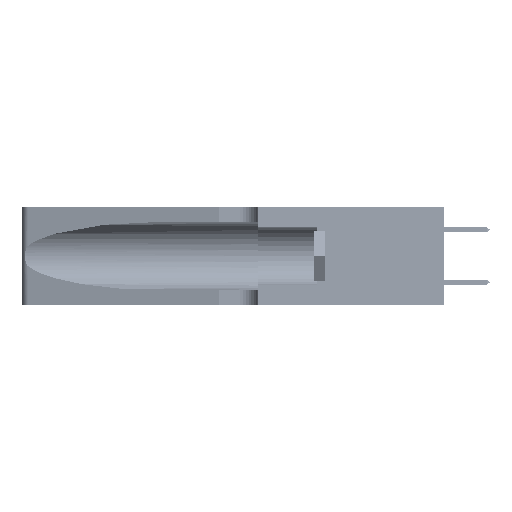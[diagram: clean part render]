
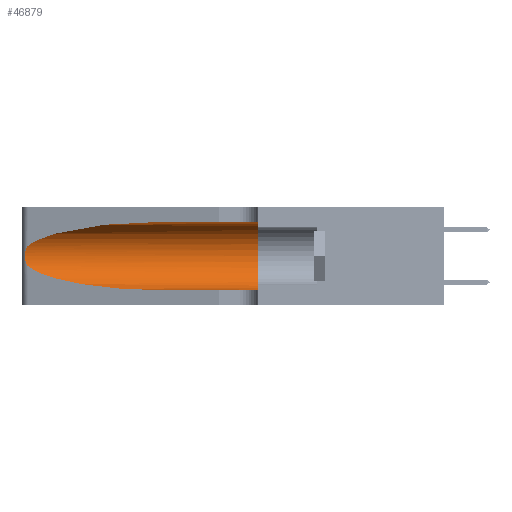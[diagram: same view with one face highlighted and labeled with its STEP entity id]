
A CAD part, left-side view. The second image highlights one B-rep face of the part: STEP entity #46879.
In plain terms, the highlighted cylindrical face has radius 3.308 mm (diameter 6.617 mm), a partial arc.
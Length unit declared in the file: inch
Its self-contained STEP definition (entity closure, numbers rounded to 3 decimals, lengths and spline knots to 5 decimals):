
#2555 = EDGE_CURVE ( 'NONE', #33973, #48274, #9177, .T. ) ;
#2716 = DIRECTION ( 'NONE',  ( 0., 1., 0. ) ) ;
#3169 = CARTESIAN_POINT ( 'NONE',  ( 0.26075, 1.23896, 0.19203 ) ) ;
#3347 = CARTESIAN_POINT ( 'NONE',  ( 0.25854, 1.2359, 0.20912 ) ) ;
#4081 = CARTESIAN_POINT ( 'NONE',  ( 0.25487, 1.22718, 0.14631 ) ) ;
#6239 = CARTESIAN_POINT ( 'NONE',  ( 0.2373, 1.15595, 0.08982 ) ) ;
#6673 = CARTESIAN_POINT ( 'NONE',  ( 0.25487, 1.22718, 0.22369 ) ) ;
#7035 = ORIENTED_EDGE ( 'NONE', *, *, #21772, .T. ) ;
#7107 = VERTEX_POINT ( 'NONE', #26929 ) ;
#7726 = CARTESIAN_POINT ( 'NONE',  ( 0.1305, 1.61858, 0.185 ) ) ;
#7785 = CARTESIAN_POINT ( 'NONE',  ( 0.25639, 1.23186, 0.15144 ) ) ;
#8476 = EDGE_CURVE ( 'NONE', #7107, #53005, #45758, .T. ) ;
#9177 = LINE ( 'NONE', #29604, #29021 ) ;
#10412 =( BOUNDED_CURVE ( )  B_SPLINE_CURVE ( 3, ( #53652, #6239, #24004, #23626 ),
 .UNSPECIFIED., .F., .F. ) 
 B_SPLINE_CURVE_WITH_KNOTS ( ( 4, 4 ),
 ( 3.44316, 4.71239 ),
 .UNSPECIFIED. ) 
 CURVE ( )  GEOMETRIC_REPRESENTATION_ITEM ( )  RATIONAL_B_SPLINE_CURVE ( ( 1., 0.87, 0.87, 1. ) ) 
 REPRESENTATION_ITEM ( '' )  );
#11701 = CARTESIAN_POINT ( 'NONE',  ( 0.25555, 1.22994, 0.2215 ) ) ;
#11815 = DIRECTION ( 'NONE',  ( 0., -1., 0. ) ) ;
#12780 = VERTEX_POINT ( 'NONE', #52701 ) ;
#13493 = DIRECTION ( 'NONE',  ( 0., -1., 0. ) ) ;
#15326 = CARTESIAN_POINT ( 'NONE',  ( 0.1305, 0.72297, 0.05475 ) ) ;
#15945 = CARTESIAN_POINT ( 'NONE',  ( 0.26017, 1.23833, 0.17102 ) ) ;
#16654 = ORIENTED_EDGE ( 'NONE', *, *, #2555, .T. ) ;
#16824 = DIRECTION ( 'NONE',  ( 0., -1., 0. ) ) ;
#18692 = EDGE_LOOP ( 'NONE', ( #21820, #38953, #7035, #16654, #36237, #28932 ) ) ;
#20392 = CARTESIAN_POINT ( 'NONE',  ( 0.25639, 1.23184, 0.21858 ) ) ;
#20568 = CARTESIAN_POINT ( 'NONE',  ( 0.25487, 1.22718, 0.14631 ) ) ;
#21772 = EDGE_CURVE ( 'NONE', #44751, #33973, #10412, .T. ) ;
#21820 = ORIENTED_EDGE ( 'NONE', *, *, #8476, .T. ) ;
#22798 = CARTESIAN_POINT ( 'NONE',  ( 0.1305, 0.72297, 0.31525 ) ) ;
#23626 = CARTESIAN_POINT ( 'NONE',  ( 0.1305, 0.72297, 0.05475 ) ) ;
#23639 = CARTESIAN_POINT ( 'NONE',  ( 0.1305, 0.35, 0.185 ) ) ;
#24004 = CARTESIAN_POINT ( 'NONE',  ( 0.18966, 0.96281, 0.05475 ) ) ;
#24282 = EDGE_CURVE ( 'NONE', #53005, #44751, #35855, .T. ) ;
#25001 = CARTESIAN_POINT ( 'NONE',  ( 0.25856, 1.23593, 0.16098 ) ) ;
#25048 = AXIS2_PLACEMENT_3D ( 'NONE', #23639, #2716, #27915 ) ;
#26258 = CARTESIAN_POINT ( 'NONE',  ( 0.1305, 1.61858, 0.31525 ) ) ;
#26929 = CARTESIAN_POINT ( 'NONE',  ( 0.1305, 0.72297, 0.31525 ) ) ;
#27426 = CARTESIAN_POINT ( 'NONE',  ( 0.2373, 1.15595, 0.28018 ) ) ;
#27789 = CARTESIAN_POINT ( 'NONE',  ( 0.18966, 0.96281, 0.31525 ) ) ;
#27915 = DIRECTION ( 'NONE',  ( 0., 0., 1. ) ) ;
#28525 = CARTESIAN_POINT ( 'NONE',  ( 0.26018, 1.23835, 0.19895 ) ) ;
#28932 = ORIENTED_EDGE ( 'NONE', *, *, #38137, .F. ) ;
#29021 = VECTOR ( 'NONE', #16824, 39.37008 ) ;
#29604 = CARTESIAN_POINT ( 'NONE',  ( 0.1305, 1.61858, 0.05475 ) ) ;
#32244 = CARTESIAN_POINT ( 'NONE',  ( 0.1305, 0.35, 0.05475 ) ) ;
#32956 = CARTESIAN_POINT ( 'NONE',  ( 0.26075, 1.23896, 0.178 ) ) ;
#33136 = CARTESIAN_POINT ( 'NONE',  ( 0.25789, 1.23486, 0.15765 ) ) ;
#33791 = AXIS2_PLACEMENT_3D ( 'NONE', #7726, #11815, #54234 ) ;
#33973 = VERTEX_POINT ( 'NONE', #15326 ) ;
#35855 = B_SPLINE_CURVE_WITH_KNOTS ( 'NONE', 3,
 ( #45423, #11701, #20392, #41677, #3347, #28525, #3169, #32956, #15945, #25001, #33136, #7785, #49654, #20568 ),
 .UNSPECIFIED., .F., .F.,
 ( 4, 2, 2, 2, 2, 2, 4 ),
 ( 0., 0.00027, 0.00053, 0.00107, 0.0016, 0.00187, 0.00214 ),
 .UNSPECIFIED. ) ;
#36237 = ORIENTED_EDGE ( 'NONE', *, *, #36419, .F. ) ;
#36419 = EDGE_CURVE ( 'NONE', #12780, #48274, #53170, .T. ) ;
#37416 = FACE_OUTER_BOUND ( 'NONE', #18692, .T. ) ;
#38137 = EDGE_CURVE ( 'NONE', #7107, #12780, #40241, .T. ) ;
#38953 = ORIENTED_EDGE ( 'NONE', *, *, #24282, .T. ) ;
#40241 = LINE ( 'NONE', #26258, #49558 ) ;
#41677 = CARTESIAN_POINT ( 'NONE',  ( 0.25787, 1.23484, 0.2124 ) ) ;
#42781 = CYLINDRICAL_SURFACE ( 'NONE', #33791, 0.13025 ) ;
#44751 = VERTEX_POINT ( 'NONE', #4081 ) ;
#45423 = CARTESIAN_POINT ( 'NONE',  ( 0.25487, 1.22718, 0.22369 ) ) ;
#45758 =( BOUNDED_CURVE ( )  B_SPLINE_CURVE ( 3, ( #22798, #27789, #27426, #6673 ),
 .UNSPECIFIED., .F., .F. ) 
 B_SPLINE_CURVE_WITH_KNOTS ( ( 4, 4 ),
 ( 1.5708, 2.84003 ),
 .UNSPECIFIED. ) 
 CURVE ( )  GEOMETRIC_REPRESENTATION_ITEM ( )  RATIONAL_B_SPLINE_CURVE ( ( 1., 0.87, 0.87, 1. ) ) 
 REPRESENTATION_ITEM ( '' )  );
#46879 = ADVANCED_FACE ( 'NONE', ( #37416 ), #42781, .F. ) ;
#48274 = VERTEX_POINT ( 'NONE', #32244 ) ;
#49558 = VECTOR ( 'NONE', #13493, 39.37008 ) ;
#49654 = CARTESIAN_POINT ( 'NONE',  ( 0.25555, 1.22993, 0.14849 ) ) ;
#49812 = CARTESIAN_POINT ( 'NONE',  ( 0.25487, 1.22718, 0.22369 ) ) ;
#52701 = CARTESIAN_POINT ( 'NONE',  ( 0.1305, 0.35, 0.31525 ) ) ;
#53005 = VERTEX_POINT ( 'NONE', #49812 ) ;
#53170 = CIRCLE ( 'NONE', #25048, 0.13025 ) ;
#53652 = CARTESIAN_POINT ( 'NONE',  ( 0.25487, 1.22718, 0.14631 ) ) ;
#54234 = DIRECTION ( 'NONE',  ( 0., 0., -1. ) ) ;
